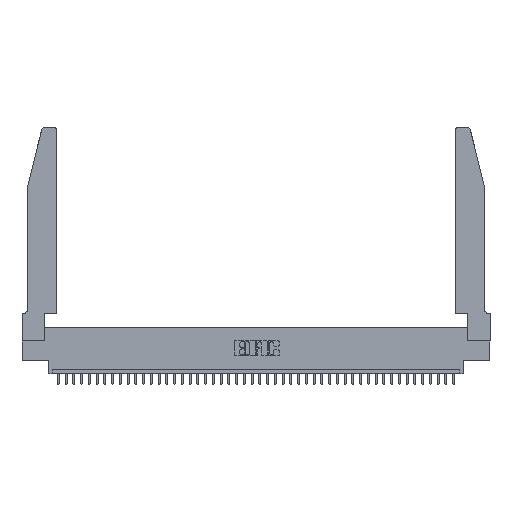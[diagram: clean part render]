
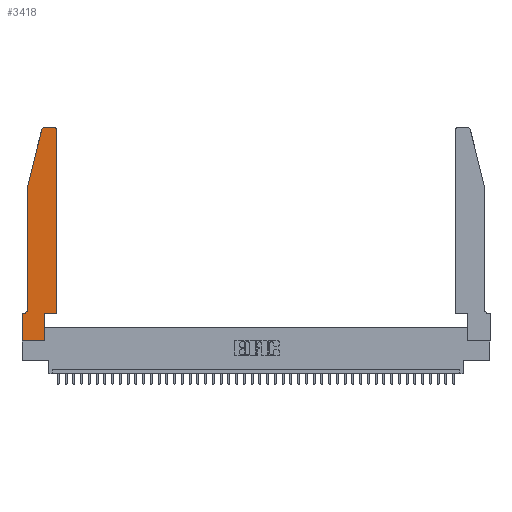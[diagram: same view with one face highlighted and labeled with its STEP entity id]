
A CAD part, top view. The second image highlights one B-rep face of the part: STEP entity #3418.
In plain terms, the highlighted planar face has unit normal (0, 0, 1).
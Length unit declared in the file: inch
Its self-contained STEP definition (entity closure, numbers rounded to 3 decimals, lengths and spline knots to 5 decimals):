
#1037 = CARTESIAN_POINT ( 'NONE',  ( 0., 0., 0.37 ) ) ;
#1305 = CARTESIAN_POINT ( 'NONE',  ( 0.4205, 2.75, 0.37 ) ) ;
#1426 = ORIENTED_EDGE ( 'NONE', *, *, #27312, .T. ) ;
#1859 = CARTESIAN_POINT ( 'NONE',  ( 0., 0., 0.37 ) ) ;
#2033 = CARTESIAN_POINT ( 'NONE',  ( 0., 0., 0.37 ) ) ;
#2461 = DIRECTION ( 'NONE',  ( -0.239, -0.971, 0. ) ) ;
#2484 = VECTOR ( 'NONE', #18261, 39.37008 ) ;
#2878 = VERTEX_POINT ( 'NONE', #38184 ) ;
#3000 = DIRECTION ( 'NONE',  ( 0., -1., 0. ) ) ;
#3395 = DIRECTION ( 'NONE',  ( 0., 0., 1. ) ) ;
#3418 = ADVANCED_FACE ( 'NONE', ( #16552 ), #22072, .T. ) ;
#3647 = VERTEX_POINT ( 'NONE', #20990 ) ;
#3679 = DIRECTION ( 'NONE',  ( 0., 1., 0. ) ) ;
#3767 = LINE ( 'NONE', #28860, #35183 ) ;
#3928 = AXIS2_PLACEMENT_3D ( 'NONE', #16055, #12890, #29260 ) ;
#4023 = LINE ( 'NONE', #1859, #25080 ) ;
#5596 = EDGE_CURVE ( 'NONE', #12112, #2878, #17860, .T. ) ;
#5908 = VERTEX_POINT ( 'NONE', #23134 ) ;
#6009 = ORIENTED_EDGE ( 'NONE', *, *, #14978, .T. ) ;
#6179 = CARTESIAN_POINT ( 'NONE',  ( 0.0755, 2., 0.37 ) ) ;
#7236 = ORIENTED_EDGE ( 'NONE', *, *, #5596, .T. ) ;
#7657 = VECTOR ( 'NONE', #3679, 39.37008 ) ;
#7781 = LINE ( 'NONE', #17594, #31994 ) ;
#9002 = DIRECTION ( 'NONE',  ( -1., 0., 0. ) ) ;
#9195 = CIRCLE ( 'NONE', #3928, 0.03 ) ;
#9390 = ORIENTED_EDGE ( 'NONE', *, *, #21129, .T. ) ;
#9685 = ORIENTED_EDGE ( 'NONE', *, *, #14722, .T. ) ;
#10177 = CARTESIAN_POINT ( 'NONE',  ( 0.2865, 0.35, 0.37 ) ) ;
#10413 = LINE ( 'NONE', #31921, #31004 ) ;
#10575 = CARTESIAN_POINT ( 'NONE',  ( 0.4505, 0.35, 0.37 ) ) ;
#10955 = CARTESIAN_POINT ( 'NONE',  ( 0.0055, 0.35, 0.37 ) ) ;
#12112 = VERTEX_POINT ( 'NONE', #1037 ) ;
#12890 = DIRECTION ( 'NONE',  ( 0., 0., 1. ) ) ;
#12910 = ORIENTED_EDGE ( 'NONE', *, *, #16750, .T. ) ;
#13492 = DIRECTION ( 'NONE',  ( 0., 1., 0. ) ) ;
#14103 = DIRECTION ( 'NONE',  ( -1., 0., 0. ) ) ;
#14499 = EDGE_LOOP ( 'NONE', ( #9685, #35523, #6009, #36981, #20130, #38070, #42185, #7236, #9390, #1426, #12910, #37520 ) ) ;
#14722 = EDGE_CURVE ( 'NONE', #28891, #15047, #28433, .T. ) ;
#14978 = EDGE_CURVE ( 'NONE', #3647, #25498, #10413, .T. ) ;
#15025 = EDGE_CURVE ( 'NONE', #25498, #5908, #21197, .T. ) ;
#15047 = VERTEX_POINT ( 'NONE', #30087 ) ;
#15485 = CARTESIAN_POINT ( 'NONE',  ( 0.4505, 0.35, 0.37 ) ) ;
#15601 = EDGE_CURVE ( 'NONE', #19019, #27688, #7781, .T. ) ;
#15691 = CIRCLE ( 'NONE', #26424, 0.03 ) ;
#16055 = CARTESIAN_POINT ( 'NONE',  ( 0.284, 2.72, 0.37 ) ) ;
#16477 = CARTESIAN_POINT ( 'NONE',  ( 0.4205, 2.72, 0.37 ) ) ;
#16552 = FACE_OUTER_BOUND ( 'NONE', #14499, .T. ) ;
#16750 = EDGE_CURVE ( 'NONE', #28859, #34769, #32892, .T. ) ;
#17594 = CARTESIAN_POINT ( 'NONE',  ( 0.0755, 0.35, 0.37 ) ) ;
#17860 = LINE ( 'NONE', #2033, #2484 ) ;
#17939 = DIRECTION ( 'NONE',  ( 0., -1., 0. ) ) ;
#18261 = DIRECTION ( 'NONE',  ( 1., 0., 0. ) ) ;
#19019 = VERTEX_POINT ( 'NONE', #10955 ) ;
#20130 = ORIENTED_EDGE ( 'NONE', *, *, #39942, .T. ) ;
#20990 = CARTESIAN_POINT ( 'NONE',  ( 0.25487, 2.72718, 0.37 ) ) ;
#21119 = CARTESIAN_POINT ( 'NONE',  ( 0.0755, 2., 0.37 ) ) ;
#21129 = EDGE_CURVE ( 'NONE', #2878, #22079, #22247, .T. ) ;
#21197 = LINE ( 'NONE', #6179, #28952 ) ;
#21599 = DIRECTION ( 'NONE',  ( 0., 0., -1. ) ) ;
#22072 = PLANE ( 'NONE',  #31510 ) ;
#22079 = VERTEX_POINT ( 'NONE', #23605 ) ;
#22247 = LINE ( 'NONE', #10177, #40329 ) ;
#22363 = CARTESIAN_POINT ( 'NONE',  ( 0., 0.35, 0.37 ) ) ;
#22794 = VECTOR ( 'NONE', #14103, 39.37008 ) ;
#23134 = CARTESIAN_POINT ( 'NONE',  ( 0.0755, 0.42, 0.37 ) ) ;
#23605 = CARTESIAN_POINT ( 'NONE',  ( 0.2865, 0.35, 0.37 ) ) ;
#24214 = EDGE_CURVE ( 'NONE', #27688, #12112, #4023, .T. ) ;
#24413 = EDGE_CURVE ( 'NONE', #15047, #3647, #9195, .T. ) ;
#25080 = VECTOR ( 'NONE', #17939, 39.37008 ) ;
#25498 = VERTEX_POINT ( 'NONE', #21119 ) ;
#26369 = DIRECTION ( 'NONE',  ( 1., 0., 0. ) ) ;
#26424 = AXIS2_PLACEMENT_3D ( 'NONE', #16477, #3395, #26369 ) ;
#27312 = EDGE_CURVE ( 'NONE', #22079, #28859, #3767, .T. ) ;
#27688 = VERTEX_POINT ( 'NONE', #34647 ) ;
#28433 = LINE ( 'NONE', #40306, #22794 ) ;
#28859 = VERTEX_POINT ( 'NONE', #15485 ) ;
#28860 = CARTESIAN_POINT ( 'NONE',  ( 0.4505, 0.35, 0.37 ) ) ;
#28891 = VERTEX_POINT ( 'NONE', #1305 ) ;
#28952 = VECTOR ( 'NONE', #3000, 39.37008 ) ;
#29128 = DIRECTION ( 'NONE',  ( 0., 0., 1. ) ) ;
#29247 = DIRECTION ( 'NONE',  ( -1., 0., 0. ) ) ;
#29260 = DIRECTION ( 'NONE',  ( 1., 0., 0. ) ) ;
#30087 = CARTESIAN_POINT ( 'NONE',  ( 0.284, 2.75, 0.37 ) ) ;
#31004 = VECTOR ( 'NONE', #2461, 39.37008 ) ;
#31510 = AXIS2_PLACEMENT_3D ( 'NONE', #22363, #29128, #32462 ) ;
#31921 = CARTESIAN_POINT ( 'NONE',  ( 0.0755, 2., 0.37 ) ) ;
#31994 = VECTOR ( 'NONE', #29247, 39.37008 ) ;
#32144 = CIRCLE ( 'NONE', #34450, 0.07 ) ;
#32462 = DIRECTION ( 'NONE',  ( 1., 0., 0. ) ) ;
#32892 = LINE ( 'NONE', #10575, #7657 ) ;
#34450 = AXIS2_PLACEMENT_3D ( 'NONE', #38647, #21599, #9002 ) ;
#34647 = CARTESIAN_POINT ( 'NONE',  ( 0., 0.35, 0.37 ) ) ;
#34769 = VERTEX_POINT ( 'NONE', #39590 ) ;
#35090 = DIRECTION ( 'NONE',  ( 1., 0., 0. ) ) ;
#35183 = VECTOR ( 'NONE', #35090, 39.37008 ) ;
#35523 = ORIENTED_EDGE ( 'NONE', *, *, #24413, .T. ) ;
#36981 = ORIENTED_EDGE ( 'NONE', *, *, #15025, .T. ) ;
#37520 = ORIENTED_EDGE ( 'NONE', *, *, #39579, .T. ) ;
#38070 = ORIENTED_EDGE ( 'NONE', *, *, #15601, .T. ) ;
#38184 = CARTESIAN_POINT ( 'NONE',  ( 0.2865, 0., 0.37 ) ) ;
#38647 = CARTESIAN_POINT ( 'NONE',  ( 0.0055, 0.42, 0.37 ) ) ;
#39579 = EDGE_CURVE ( 'NONE', #34769, #28891, #15691, .T. ) ;
#39590 = CARTESIAN_POINT ( 'NONE',  ( 0.4505, 2.72, 0.37 ) ) ;
#39942 = EDGE_CURVE ( 'NONE', #5908, #19019, #32144, .T. ) ;
#40306 = CARTESIAN_POINT ( 'NONE',  ( 0.2605, 2.75, 0.37 ) ) ;
#40329 = VECTOR ( 'NONE', #13492, 39.37008 ) ;
#42185 = ORIENTED_EDGE ( 'NONE', *, *, #24214, .T. ) ;
